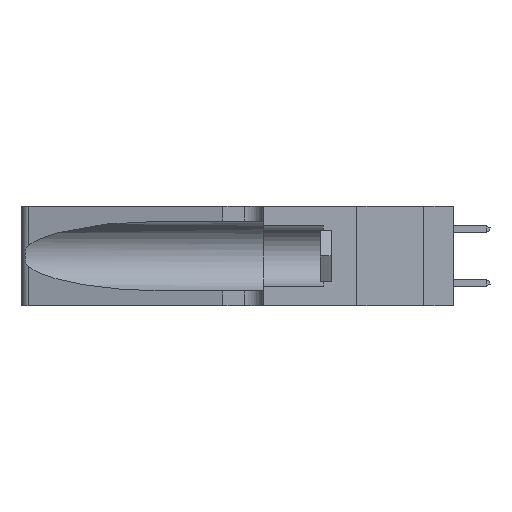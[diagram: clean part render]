
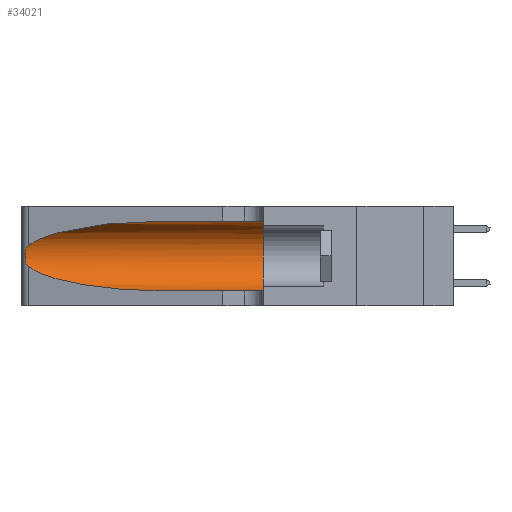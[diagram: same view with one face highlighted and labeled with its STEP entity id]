
A CAD part, left-side view. The second image highlights one B-rep face of the part: STEP entity #34021.
In plain terms, the highlighted cylindrical face has radius 3.308 mm (diameter 6.617 mm), a partial arc.
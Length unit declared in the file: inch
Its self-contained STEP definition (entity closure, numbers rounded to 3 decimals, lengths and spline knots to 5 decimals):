
#53 = EDGE_CURVE ( 'NONE', #16850, #21626, #11463, .T. ) ;
#1378 = CARTESIAN_POINT ( 'NONE',  ( 0.25555, 1.22993, 0.14849 ) ) ;
#1404 = CIRCLE ( 'NONE', #37264, 0.13025 ) ;
#1512 = CARTESIAN_POINT ( 'NONE',  ( 0.1305, 1.61858, 0.05475 ) ) ;
#2635 = CARTESIAN_POINT ( 'NONE',  ( 0.1305, 0.35, 0.31525 ) ) ;
#2881 = CARTESIAN_POINT ( 'NONE',  ( 0.2373, 1.15595, 0.28018 ) ) ;
#3047 = CARTESIAN_POINT ( 'NONE',  ( 0.25854, 1.2359, 0.20912 ) ) ;
#4223 = CARTESIAN_POINT ( 'NONE',  ( 0.25487, 1.22718, 0.14631 ) ) ;
#4649 = CARTESIAN_POINT ( 'NONE',  ( 0.1305, 0.72297, 0.05475 ) ) ;
#5537 = ORIENTED_EDGE ( 'NONE', *, *, #34930, .F. ) ;
#5776 =( BOUNDED_CURVE ( )  B_SPLINE_CURVE ( 3, ( #14163, #23218, #16985, #4649 ),
 .UNSPECIFIED., .F., .T. ) 
 B_SPLINE_CURVE_WITH_KNOTS ( ( 4, 4 ),
 ( 3.44316, 4.71239 ),
 .UNSPECIFIED. ) 
 CURVE ( )  GEOMETRIC_REPRESENTATION_ITEM ( )  RATIONAL_B_SPLINE_CURVE ( ( 1., 0.87, 0.87, 1. ) ) 
 REPRESENTATION_ITEM ( '' )  );
#7164 = CARTESIAN_POINT ( 'NONE',  ( 0.26075, 1.23896, 0.178 ) ) ;
#7429 = CARTESIAN_POINT ( 'NONE',  ( 0.26017, 1.23833, 0.17102 ) ) ;
#8446 = DIRECTION ( 'NONE',  ( 0., 1., 0. ) ) ;
#8721 = CARTESIAN_POINT ( 'NONE',  ( 0.1305, 0.72297, 0.31525 ) ) ;
#8912 = ORIENTED_EDGE ( 'NONE', *, *, #53, .T. ) ;
#9075 = VECTOR ( 'NONE', #19929, 39.37008 ) ;
#9458 = EDGE_CURVE ( 'NONE', #34783, #20909, #15096, .T. ) ;
#9553 = CARTESIAN_POINT ( 'NONE',  ( 0.1305, 0.72297, 0.05475 ) ) ;
#11463 = LINE ( 'NONE', #1512, #9075 ) ;
#12333 = DIRECTION ( 'NONE',  ( 0., -1., 0. ) ) ;
#12808 = VERTEX_POINT ( 'NONE', #2635 ) ;
#13065 = ORIENTED_EDGE ( 'NONE', *, *, #23259, .F. ) ;
#14163 = CARTESIAN_POINT ( 'NONE',  ( 0.25487, 1.22718, 0.14631 ) ) ;
#15096 = B_SPLINE_CURVE_WITH_KNOTS ( 'NONE', 3,
 ( #25139, #32149, #15356, #15481, #3047, #25488, #35039, #7164, #7429, #19682, #19544, #29007, #1378, #4223 ),
 .UNSPECIFIED., .F., .F.,
 ( 4, 2, 2, 2, 2, 2, 4 ),
 ( 0., 0.00027, 0.00053, 0.00107, 0.0016, 0.00187, 0.00214 ),
 .UNSPECIFIED. ) ;
#15356 = CARTESIAN_POINT ( 'NONE',  ( 0.25639, 1.23184, 0.21858 ) ) ;
#15481 = CARTESIAN_POINT ( 'NONE',  ( 0.25787, 1.23484, 0.2124 ) ) ;
#16850 = VERTEX_POINT ( 'NONE', #9553 ) ;
#16985 = CARTESIAN_POINT ( 'NONE',  ( 0.18966, 0.96281, 0.05475 ) ) ;
#17162 = DIRECTION ( 'NONE',  ( 0., 0., 1. ) ) ;
#19544 = CARTESIAN_POINT ( 'NONE',  ( 0.25789, 1.23486, 0.15765 ) ) ;
#19682 = CARTESIAN_POINT ( 'NONE',  ( 0.25856, 1.23593, 0.16098 ) ) ;
#19798 = EDGE_CURVE ( 'NONE', #29960, #34783, #34380, .T. ) ;
#19929 = DIRECTION ( 'NONE',  ( 0., -1., 0. ) ) ;
#20909 = VERTEX_POINT ( 'NONE', #26306 ) ;
#21285 = CARTESIAN_POINT ( 'NONE',  ( 0.1305, 0.72297, 0.31525 ) ) ;
#21626 = VERTEX_POINT ( 'NONE', #31000 ) ;
#21727 = AXIS2_PLACEMENT_3D ( 'NONE', #34123, #12333, #30785 ) ;
#22168 = CYLINDRICAL_SURFACE ( 'NONE', #21727, 0.13025 ) ;
#22910 = ORIENTED_EDGE ( 'NONE', *, *, #19798, .T. ) ;
#23218 = CARTESIAN_POINT ( 'NONE',  ( 0.2373, 1.15595, 0.08982 ) ) ;
#23259 = EDGE_CURVE ( 'NONE', #29960, #12808, #30022, .T. ) ;
#24252 = VECTOR ( 'NONE', #27793, 39.37008 ) ;
#24393 = ORIENTED_EDGE ( 'NONE', *, *, #28525, .T. ) ;
#24685 = CARTESIAN_POINT ( 'NONE',  ( 0.1305, 1.61858, 0.31525 ) ) ;
#25139 = CARTESIAN_POINT ( 'NONE',  ( 0.25487, 1.22718, 0.22369 ) ) ;
#25488 = CARTESIAN_POINT ( 'NONE',  ( 0.26018, 1.23835, 0.19895 ) ) ;
#25958 = EDGE_LOOP ( 'NONE', ( #22910, #37081, #24393, #8912, #5537, #13065 ) ) ;
#26306 = CARTESIAN_POINT ( 'NONE',  ( 0.25487, 1.22718, 0.14631 ) ) ;
#27793 = DIRECTION ( 'NONE',  ( 0., -1., 0. ) ) ;
#28525 = EDGE_CURVE ( 'NONE', #20909, #16850, #5776, .T. ) ;
#28828 = CARTESIAN_POINT ( 'NONE',  ( 0.25487, 1.22718, 0.22369 ) ) ;
#29007 = CARTESIAN_POINT ( 'NONE',  ( 0.25639, 1.23186, 0.15144 ) ) ;
#29960 = VERTEX_POINT ( 'NONE', #8721 ) ;
#29989 = CARTESIAN_POINT ( 'NONE',  ( 0.1305, 0.35, 0.185 ) ) ;
#30022 = LINE ( 'NONE', #24685, #24252 ) ;
#30176 = CARTESIAN_POINT ( 'NONE',  ( 0.18966, 0.96281, 0.31525 ) ) ;
#30463 = CARTESIAN_POINT ( 'NONE',  ( 0.25487, 1.22718, 0.22369 ) ) ;
#30785 = DIRECTION ( 'NONE',  ( 0., 0., -1. ) ) ;
#31000 = CARTESIAN_POINT ( 'NONE',  ( 0.1305, 0.35, 0.05475 ) ) ;
#32149 = CARTESIAN_POINT ( 'NONE',  ( 0.25555, 1.22994, 0.2215 ) ) ;
#32768 = FACE_OUTER_BOUND ( 'NONE', #25958, .T. ) ;
#34021 = ADVANCED_FACE ( 'NONE', ( #32768 ), #22168, .F. ) ;
#34123 = CARTESIAN_POINT ( 'NONE',  ( 0.1305, 1.61858, 0.185 ) ) ;
#34380 =( BOUNDED_CURVE ( )  B_SPLINE_CURVE ( 3, ( #21285, #30176, #2881, #30463 ),
 .UNSPECIFIED., .F., .F. ) 
 B_SPLINE_CURVE_WITH_KNOTS ( ( 4, 4 ),
 ( 1.5708, 2.84003 ),
 .UNSPECIFIED. ) 
 CURVE ( )  GEOMETRIC_REPRESENTATION_ITEM ( )  RATIONAL_B_SPLINE_CURVE ( ( 1., 0.87, 0.87, 1. ) ) 
 REPRESENTATION_ITEM ( '' )  );
#34783 = VERTEX_POINT ( 'NONE', #28828 ) ;
#34930 = EDGE_CURVE ( 'NONE', #12808, #21626, #1404, .T. ) ;
#35039 = CARTESIAN_POINT ( 'NONE',  ( 0.26075, 1.23896, 0.19203 ) ) ;
#37081 = ORIENTED_EDGE ( 'NONE', *, *, #9458, .T. ) ;
#37264 = AXIS2_PLACEMENT_3D ( 'NONE', #29989, #8446, #17162 ) ;
